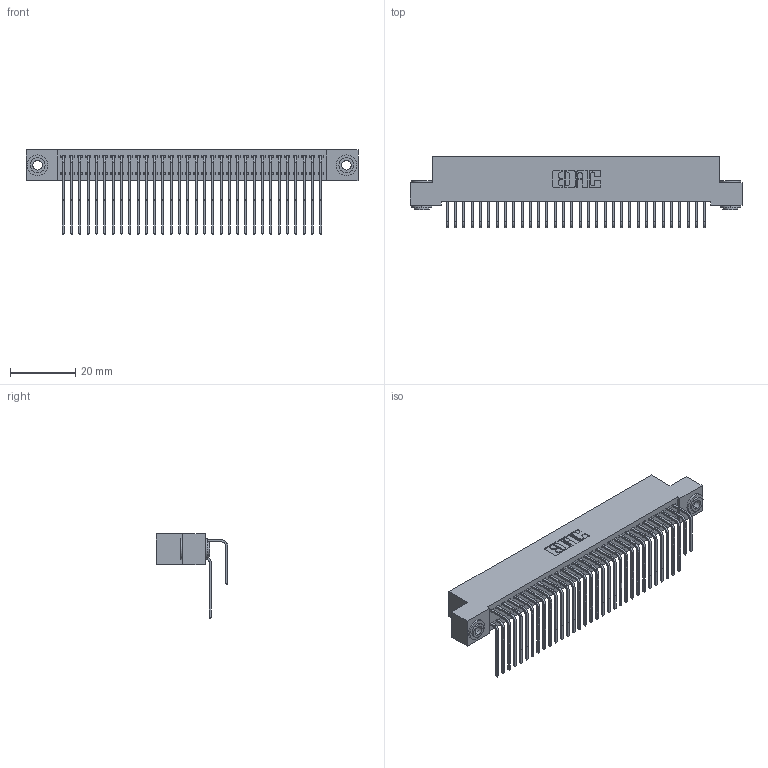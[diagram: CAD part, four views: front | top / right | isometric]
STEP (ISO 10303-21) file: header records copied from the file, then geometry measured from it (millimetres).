
FILE_DESCRIPTION (( 'STEP AP203' ), '1' );
FILE_NAME ('342-064-558-203.STEP', '2019-10-03T14:35:46', ( '' ), ( '' ), 'SwSTEP 2.0', 'SolidWorks 2016', '' );
FILE_SCHEMA (( 'CONFIG_CONTROL_DESIGN' ));
Length unit declared in the file: inch
Products named in the file (5): 342-250-002_345-250-002-102; 342-064-558-203; 342 Part_.156 TH; 345-292-001_558 559 Tail - 1; 345-292-001_558 Tail - 2
Assembly tree (67 placements, depth 2):
  342-064-558-203
    342 Part_.156 TH
    345-292-001_558 559 Tail - 1  x32
    345-292-001_558 Tail - 2  x32
    342-250-002_345-250-002-102  x2
Bounding box: 101.6 x 21.91 x 25.78 mm (x, y, z)
Volume: 9473.4 mm3; surface area: 17058.2 mm2
Topology: 67 solids, 67 shells, 3604 faces, 10679 edges, 7030 vertices
Faces by surface type: plane 2508, cylinder 1088, cone 8
Entity records: 24182 total; most frequent: CARTESIAN_POINT 4044, ORIENTED_EDGE 3922, DIRECTION 3487, EDGE_CURVE 1961, VECTOR 1769, LINE 1769, VERTEX_POINT 1302, AXIS2_PLACEMENT_3D 859
